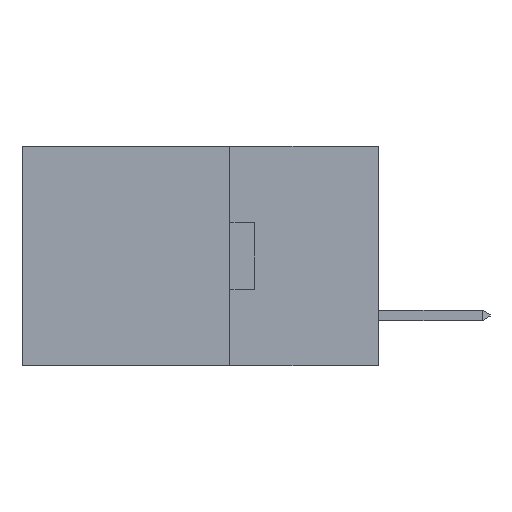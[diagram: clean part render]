
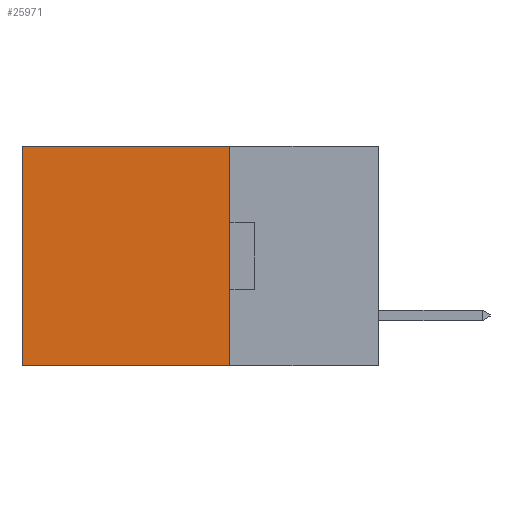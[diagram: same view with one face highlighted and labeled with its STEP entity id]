
A CAD part, left-side view. The second image highlights one B-rep face of the part: STEP entity #25971.
In plain terms, the highlighted planar face has unit normal (-1, 0, 0).
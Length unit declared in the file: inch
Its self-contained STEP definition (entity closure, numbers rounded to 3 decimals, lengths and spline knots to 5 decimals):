
#662 = CARTESIAN_POINT ( 'NONE',  ( 0.2615, 0.6, -0.37 ) ) ;
#668 = DIRECTION ( 'NONE',  ( 0., 0., -1. ) ) ;
#1330 = PLANE ( 'NONE',  #14902 ) ;
#1552 = VERTEX_POINT ( 'NONE', #5926 ) ;
#3541 = DIRECTION ( 'NONE',  ( 0., 0., -1. ) ) ;
#4809 = ORIENTED_EDGE ( 'NONE', *, *, #5365, .F. ) ;
#5184 = EDGE_CURVE ( 'NONE', #17423, #1552, #6794, .T. ) ;
#5365 = EDGE_CURVE ( 'NONE', #27067, #21215, #9179, .T. ) ;
#5926 = CARTESIAN_POINT ( 'NONE',  ( 0.2615, 0.6, -0.37 ) ) ;
#6786 = LINE ( 'NONE', #26579, #23008 ) ;
#6794 = LINE ( 'NONE', #662, #23658 ) ;
#9147 = CARTESIAN_POINT ( 'NONE',  ( 0.2615, 0.25, 0. ) ) ;
#9179 = LINE ( 'NONE', #14108, #19769 ) ;
#9472 = VECTOR ( 'NONE', #10182, 39.37008 ) ;
#10107 = ORIENTED_EDGE ( 'NONE', *, *, #16810, .F. ) ;
#10182 = DIRECTION ( 'NONE',  ( 0., 1., 0. ) ) ;
#10195 = ORIENTED_EDGE ( 'NONE', *, *, #5184, .T. ) ;
#11867 = DIRECTION ( 'NONE',  ( 0., 1., 0. ) ) ;
#14018 = DIRECTION ( 'NONE',  ( 0., 0., -1. ) ) ;
#14108 = CARTESIAN_POINT ( 'NONE',  ( 0.2615, 0.25, -0.37 ) ) ;
#14902 = AXIS2_PLACEMENT_3D ( 'NONE', #22531, #16289, #3541 ) ;
#15432 = EDGE_LOOP ( 'NONE', ( #10195, #10107, #4809, #16715 ) ) ;
#15682 = FACE_OUTER_BOUND ( 'NONE', #15432, .T. ) ;
#16289 = DIRECTION ( 'NONE',  ( 1., 0., 0. ) ) ;
#16715 = ORIENTED_EDGE ( 'NONE', *, *, #21779, .T. ) ;
#16810 = EDGE_CURVE ( 'NONE', #21215, #1552, #6786, .T. ) ;
#17423 = VERTEX_POINT ( 'NONE', #26356 ) ;
#19389 = LINE ( 'NONE', #22842, #9472 ) ;
#19769 = VECTOR ( 'NONE', #14018, 39.37008 ) ;
#21215 = VERTEX_POINT ( 'NONE', #22089 ) ;
#21779 = EDGE_CURVE ( 'NONE', #27067, #17423, #19389, .T. ) ;
#22089 = CARTESIAN_POINT ( 'NONE',  ( 0.2615, 0.25, -0.37 ) ) ;
#22531 = CARTESIAN_POINT ( 'NONE',  ( 0.2615, 0.25, -0.37 ) ) ;
#22842 = CARTESIAN_POINT ( 'NONE',  ( 0.2615, 0.25, 0. ) ) ;
#23008 = VECTOR ( 'NONE', #11867, 39.37008 ) ;
#23658 = VECTOR ( 'NONE', #668, 39.37008 ) ;
#25971 = ADVANCED_FACE ( 'NONE', ( #15682 ), #1330, .F. ) ;
#26356 = CARTESIAN_POINT ( 'NONE',  ( 0.2615, 0.6, 0. ) ) ;
#26579 = CARTESIAN_POINT ( 'NONE',  ( 0.2615, 0.25, -0.37 ) ) ;
#27067 = VERTEX_POINT ( 'NONE', #9147 ) ;
